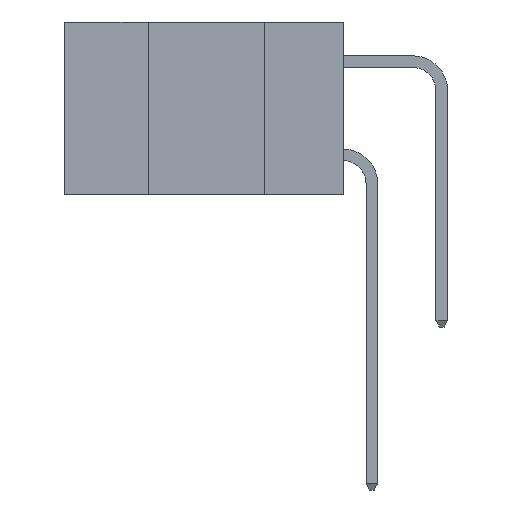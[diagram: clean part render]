
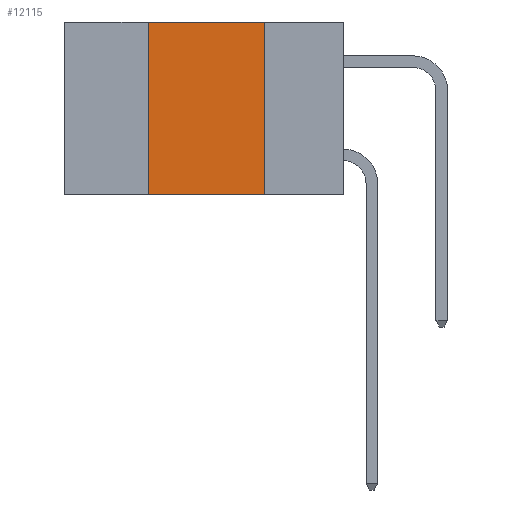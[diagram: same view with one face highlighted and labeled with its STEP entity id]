
A CAD part, left-side view. The second image highlights one B-rep face of the part: STEP entity #12115.
In plain terms, the highlighted planar face has unit normal (-1, 0, 0).
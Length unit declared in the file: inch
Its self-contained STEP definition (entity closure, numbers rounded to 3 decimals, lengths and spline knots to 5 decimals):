
#82 = CARTESIAN_POINT ( 'NONE',  ( 0., 0.17, -0.37 ) ) ;
#928 = CARTESIAN_POINT ( 'NONE',  ( 0., 0.17, -0.37 ) ) ;
#1935 = ORIENTED_EDGE ( 'NONE', *, *, #16167, .T. ) ;
#2935 = ORIENTED_EDGE ( 'NONE', *, *, #8966, .F. ) ;
#3350 = ORIENTED_EDGE ( 'NONE', *, *, #7949, .F. ) ;
#3619 = ORIENTED_EDGE ( 'NONE', *, *, #13871, .F. ) ;
#5887 = DIRECTION ( 'NONE',  ( 1., 0., 0. ) ) ;
#6005 = LINE ( 'NONE', #6888, #7299 ) ;
#6742 = FACE_OUTER_BOUND ( 'NONE', #8510, .T. ) ;
#6780 = DIRECTION ( 'NONE',  ( 0., -1., 0. ) ) ;
#6888 = CARTESIAN_POINT ( 'NONE',  ( 0., 0.42, -0.37 ) ) ;
#7022 = DIRECTION ( 'NONE',  ( 0., 0., -1. ) ) ;
#7299 = VECTOR ( 'NONE', #20079, 39.37008 ) ;
#7746 = VECTOR ( 'NONE', #6780, 39.37008 ) ;
#7949 = EDGE_CURVE ( 'NONE', #14201, #9955, #6005, .T. ) ;
#8510 = EDGE_LOOP ( 'NONE', ( #2935, #3619, #3350, #1935 ) ) ;
#8631 = DIRECTION ( 'NONE',  ( 0., -1., 0. ) ) ;
#8966 = EDGE_CURVE ( 'NONE', #9138, #9210, #20993, .T. ) ;
#9108 = AXIS2_PLACEMENT_3D ( 'NONE', #15924, #5887, #17554 ) ;
#9138 = VERTEX_POINT ( 'NONE', #20906 ) ;
#9210 = VERTEX_POINT ( 'NONE', #928 ) ;
#9955 = VERTEX_POINT ( 'NONE', #18085 ) ;
#11820 = CARTESIAN_POINT ( 'NONE',  ( 0., 0.6, 0. ) ) ;
#12115 = ADVANCED_FACE ( 'NONE', ( #6742 ), #20769, .F. ) ;
#13356 = VECTOR ( 'NONE', #7022, 39.37008 ) ;
#13871 = EDGE_CURVE ( 'NONE', #9955, #9138, #16594, .T. ) ;
#14201 = VERTEX_POINT ( 'NONE', #20694 ) ;
#15905 = VECTOR ( 'NONE', #8631, 39.37008 ) ;
#15924 = CARTESIAN_POINT ( 'NONE',  ( 0., 0.6, 0. ) ) ;
#16167 = EDGE_CURVE ( 'NONE', #14201, #9210, #20233, .T. ) ;
#16594 = LINE ( 'NONE', #11820, #7746 ) ;
#17554 = DIRECTION ( 'NONE',  ( 0., 0., -1. ) ) ;
#18085 = CARTESIAN_POINT ( 'NONE',  ( 0., 0.42, 0. ) ) ;
#20079 = DIRECTION ( 'NONE',  ( 0., 0., 1. ) ) ;
#20233 = LINE ( 'NONE', #21710, #15905 ) ;
#20694 = CARTESIAN_POINT ( 'NONE',  ( 0., 0.42, -0.37 ) ) ;
#20769 = PLANE ( 'NONE',  #9108 ) ;
#20906 = CARTESIAN_POINT ( 'NONE',  ( 0., 0.17, 0. ) ) ;
#20993 = LINE ( 'NONE', #82, #13356 ) ;
#21710 = CARTESIAN_POINT ( 'NONE',  ( 0., 0.6, -0.37 ) ) ;
